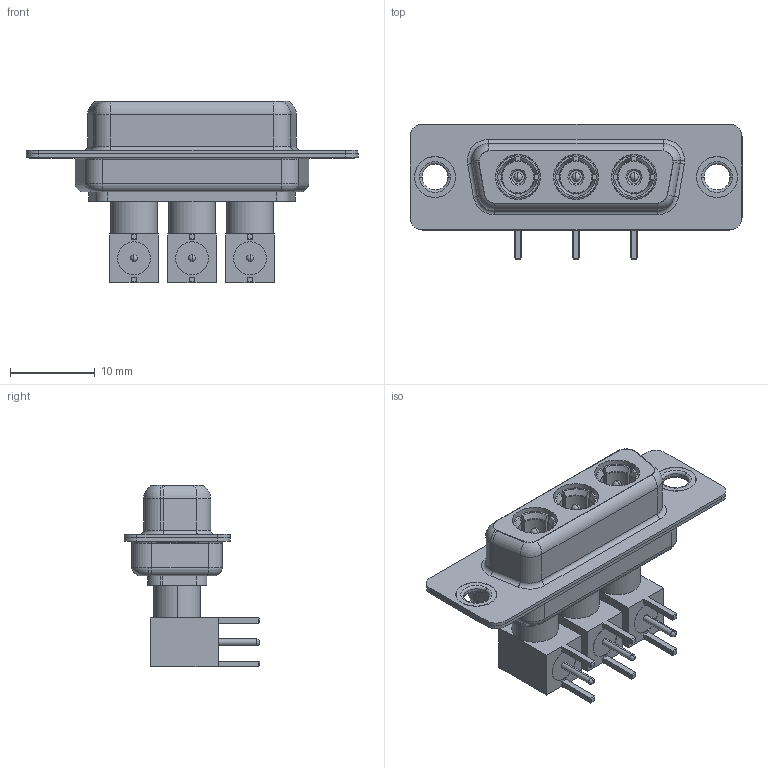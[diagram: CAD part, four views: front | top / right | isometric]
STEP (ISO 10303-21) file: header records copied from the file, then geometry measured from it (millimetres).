
FILE_DESCRIPTION (( 'STEP AP203' ), '1' );
FILE_NAME ('630-3W3-640-7N1.STEP', '2022-05-30T14:01:01', ( '' ), ( '' ), 'SwSTEP 2.0', 'SolidWorks 2020', '' );
FILE_SCHEMA (( 'CONFIG_CONTROL_DESIGN' ));
Length unit declared in the file: millimetre
Products named in the file (14): Co-Ax Plug Assy_RA; 630Combo Thru Hole Rivet; Insulator Pin_Straight PC Tail; Locking Collar; 630Combo Shell Rear_15 Contacts; 630Combo Shell Front_15 Contacts; Insulator RA Pin; 630Combo Housing_3W3; Pin_RA; RA Back Shell; 630-3W3-640-7N1; Co-Ax Plug_RA PC Tail
Assembly tree (26 placements, depth 3):
  630-3W3-640-7N1
    630Combo Housing_3W3
    630Combo Shell Front_15 Contacts
    630Combo Shell Rear_15 Contacts
    630Combo Thru Hole Rivet  x2
    Co-Ax Plug Assy_RA
      Co-Ax Plug_RA PC Tail
      Insulator Pin_Straight PC Tail
      Pin_RA
      Locking Collar
      RA Back Shell
      Insulator RA Pin
    Co-Ax Plug Assy_RA
      Co-Ax Plug_RA PC Tail
      Insulator Pin_Straight PC Tail
      Pin_RA
      Locking Collar
      RA Back Shell
      Insulator RA Pin
    Co-Ax Plug Assy_RA
      Co-Ax Plug_RA PC Tail
      Insulator Pin_Straight PC Tail
      Pin_RA
      Locking Collar
      RA Back Shell
      Insulator RA Pin
Bounding box: 39.2 x 16 x 21.41 mm (x, y, z)
Volume: 3062.3 mm3; surface area: 7644.1 mm2
Topology: 23 solids, 23 shells, 757 faces, 1806 edges, 1124 vertices
Faces by surface type: cylinder 316, plane 268, torus 83, cone 75, sphere 12, bspline 3
Entity records: 14189 total; most frequent: CARTESIAN_POINT 2460, DIRECTION 2265, ORIENTED_EDGE 1952, EDGE_CURVE 976, AXIS2_PLACEMENT_3D 918, VERTEX_POINT 612, CIRCLE 476, EDGE_LOOP 466
